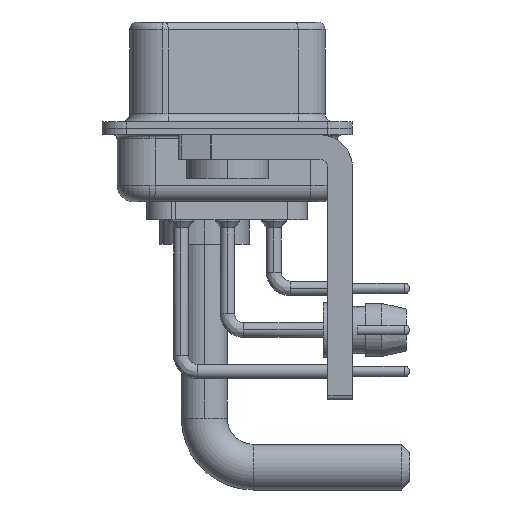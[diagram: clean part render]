
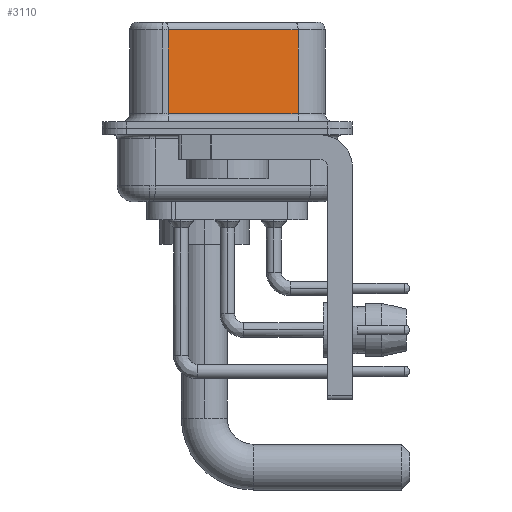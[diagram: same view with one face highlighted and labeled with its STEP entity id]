
A CAD part, left-side view. The second image highlights one B-rep face of the part: STEP entity #3110.
In plain terms, the highlighted planar face has unit normal (-0.985, -0.174, 0).
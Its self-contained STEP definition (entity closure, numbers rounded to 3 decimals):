
#42 = CARTESIAN_POINT ( 'NONE',  ( 3.73, 3.628, 6.02 ) ) ;
#861 = VECTOR ( 'NONE', #38472, 1000. ) ;
#1048 = VERTEX_POINT ( 'NONE', #42 ) ;
#2176 = DIRECTION ( 'NONE',  ( -0.174, 0.985, 0. ) ) ;
#2377 = FACE_OUTER_BOUND ( 'NONE', #24276, .T. ) ;
#3110 = ADVANCED_FACE ( 'NONE', ( #2377 ), #5715, .F. ) ;
#3641 = DIRECTION ( 'NONE',  ( 0., 0., -1. ) ) ;
#5072 = EDGE_CURVE ( 'NONE', #22401, #21564, #26286, .T. ) ;
#5715 = PLANE ( 'NONE',  #38322 ) ;
#5838 = CARTESIAN_POINT ( 'NONE',  ( 5.132, -4.322, 0.9 ) ) ;
#9744 = LINE ( 'NONE', #15448, #18159 ) ;
#11229 = ORIENTED_EDGE ( 'NONE', *, *, #20009, .F. ) ;
#11694 = VECTOR ( 'NONE', #13834, 1000. ) ;
#13497 = VERTEX_POINT ( 'NONE', #25400 ) ;
#13834 = DIRECTION ( 'NONE',  ( 0., 0., -1. ) ) ;
#15448 = CARTESIAN_POINT ( 'NONE',  ( 5.132, -4.322, 6.02 ) ) ;
#15607 = LINE ( 'NONE', #24631, #23985 ) ;
#15977 = ORIENTED_EDGE ( 'NONE', *, *, #33759, .T. ) ;
#17613 = EDGE_CURVE ( 'NONE', #13497, #1048, #9744, .T. ) ;
#18159 = VECTOR ( 'NONE', #24663, 1000. ) ;
#19710 = CARTESIAN_POINT ( 'NONE',  ( 5.132, -4.322, 6.52 ) ) ;
#20009 = EDGE_CURVE ( 'NONE', #13497, #21564, #25218, .T. ) ;
#20423 = CARTESIAN_POINT ( 'NONE',  ( 3.73, 3.628, 0.9 ) ) ;
#21564 = VERTEX_POINT ( 'NONE', #5838 ) ;
#22401 = VERTEX_POINT ( 'NONE', #20423 ) ;
#23985 = VECTOR ( 'NONE', #3641, 1000. ) ;
#24276 = EDGE_LOOP ( 'NONE', ( #11229, #35491, #15977, #35085 ) ) ;
#24631 = CARTESIAN_POINT ( 'NONE',  ( 3.73, 3.628, 6.52 ) ) ;
#24663 = DIRECTION ( 'NONE',  ( -0.174, 0.985, 0. ) ) ;
#25218 = LINE ( 'NONE', #19710, #11694 ) ;
#25400 = CARTESIAN_POINT ( 'NONE',  ( 5.132, -4.322, 6.02 ) ) ;
#26286 = LINE ( 'NONE', #29413, #861 ) ;
#26321 = DIRECTION ( 'NONE',  ( 0.985, 0.174, 0. ) ) ;
#29413 = CARTESIAN_POINT ( 'NONE',  ( 5.132, -4.322, 0.9 ) ) ;
#33759 = EDGE_CURVE ( 'NONE', #1048, #22401, #15607, .T. ) ;
#35085 = ORIENTED_EDGE ( 'NONE', *, *, #5072, .T. ) ;
#35491 = ORIENTED_EDGE ( 'NONE', *, *, #17613, .T. ) ;
#37935 = CARTESIAN_POINT ( 'NONE',  ( 5.132, -4.322, 6.52 ) ) ;
#38322 = AXIS2_PLACEMENT_3D ( 'NONE', #37935, #26321, #2176 ) ;
#38472 = DIRECTION ( 'NONE',  ( 0.174, -0.985, 0. ) ) ;
